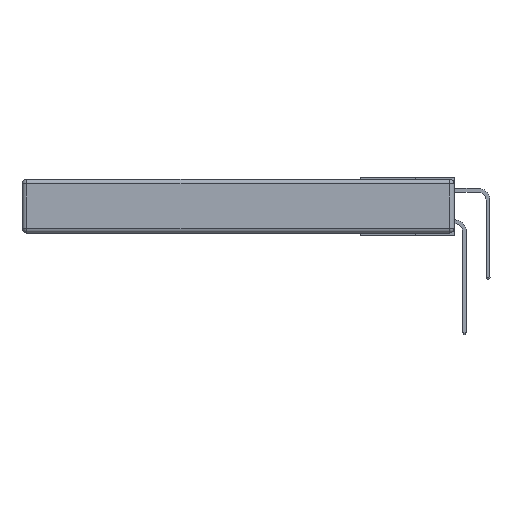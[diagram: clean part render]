
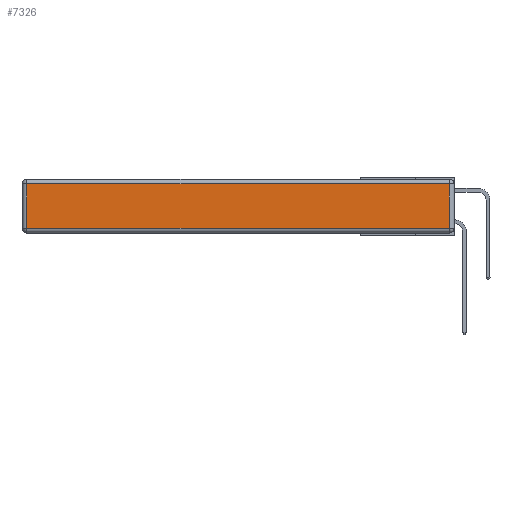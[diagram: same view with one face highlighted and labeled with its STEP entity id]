
A CAD part, left-side view. The second image highlights one B-rep face of the part: STEP entity #7326.
In plain terms, the highlighted planar face has unit normal (-1, 0, 0).
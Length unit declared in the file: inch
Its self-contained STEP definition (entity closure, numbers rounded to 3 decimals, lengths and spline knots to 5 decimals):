
#521 = DIRECTION ( 'NONE',  ( 0., 0., 1. ) ) ;
#2378 = VECTOR ( 'NONE', #5391, 39.37008 ) ;
#5391 = DIRECTION ( 'NONE',  ( 0., -1., 0. ) ) ;
#5484 = CARTESIAN_POINT ( 'NONE',  ( 0., 2.72, -0.313 ) ) ;
#6334 = ORIENTED_EDGE ( 'NONE', *, *, #6354, .T. ) ;
#6354 = EDGE_CURVE ( 'NONE', #7905, #16774, #23158, .T. ) ;
#6706 = CARTESIAN_POINT ( 'NONE',  ( 0., 0.03, -0.343 ) ) ;
#7326 = ADVANCED_FACE ( 'NONE', ( #11150 ), #24956, .T. ) ;
#7905 = VERTEX_POINT ( 'NONE', #17340 ) ;
#8834 = VECTOR ( 'NONE', #15575, 39.37008 ) ;
#9270 = VECTOR ( 'NONE', #15241, 39.37008 ) ;
#10055 = AXIS2_PLACEMENT_3D ( 'NONE', #18902, #12768, #521 ) ;
#10620 = CARTESIAN_POINT ( 'NONE',  ( 0., 2.72, -0.03 ) ) ;
#10790 = VERTEX_POINT ( 'NONE', #5484 ) ;
#11150 = FACE_OUTER_BOUND ( 'NONE', #15112, .T. ) ;
#11441 = LINE ( 'NONE', #23964, #2378 ) ;
#11497 = EDGE_CURVE ( 'NONE', #16774, #17472, #16839, .T. ) ;
#12768 = DIRECTION ( 'NONE',  ( -1., 0., 0. ) ) ;
#15112 = EDGE_LOOP ( 'NONE', ( #22202, #6334, #22318, #20010 ) ) ;
#15232 = EDGE_CURVE ( 'NONE', #17472, #10790, #25670, .T. ) ;
#15241 = DIRECTION ( 'NONE',  ( 0., 0., 1. ) ) ;
#15575 = DIRECTION ( 'NONE',  ( 0., 0., -1. ) ) ;
#16429 = CARTESIAN_POINT ( 'NONE',  ( 0., 2.75, -0.03 ) ) ;
#16774 = VERTEX_POINT ( 'NONE', #26628 ) ;
#16839 = LINE ( 'NONE', #16429, #21037 ) ;
#17340 = CARTESIAN_POINT ( 'NONE',  ( 0., 0.03, -0.313 ) ) ;
#17472 = VERTEX_POINT ( 'NONE', #10620 ) ;
#18477 = DIRECTION ( 'NONE',  ( 0., 1., 0. ) ) ;
#18902 = CARTESIAN_POINT ( 'NONE',  ( 0., 0., -0.343 ) ) ;
#20010 = ORIENTED_EDGE ( 'NONE', *, *, #15232, .T. ) ;
#21037 = VECTOR ( 'NONE', #18477, 39.37008 ) ;
#21454 = EDGE_CURVE ( 'NONE', #10790, #7905, #11441, .T. ) ;
#22202 = ORIENTED_EDGE ( 'NONE', *, *, #21454, .T. ) ;
#22318 = ORIENTED_EDGE ( 'NONE', *, *, #11497, .T. ) ;
#23158 = LINE ( 'NONE', #6706, #9270 ) ;
#23828 = CARTESIAN_POINT ( 'NONE',  ( 0., 2.72, -0.343 ) ) ;
#23964 = CARTESIAN_POINT ( 'NONE',  ( 0., 0., -0.313 ) ) ;
#24956 = PLANE ( 'NONE',  #10055 ) ;
#25670 = LINE ( 'NONE', #23828, #8834 ) ;
#26628 = CARTESIAN_POINT ( 'NONE',  ( 0., 0.03, -0.03 ) ) ;
